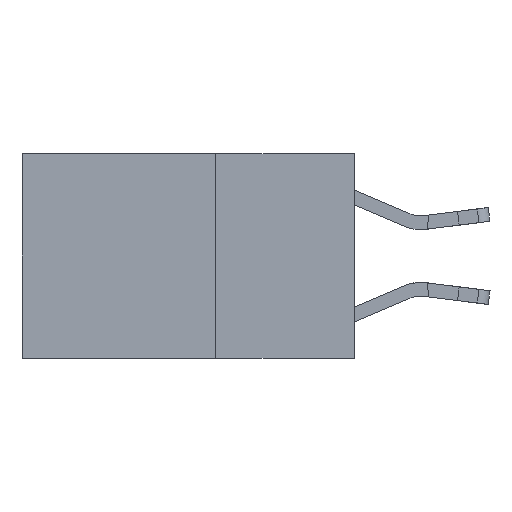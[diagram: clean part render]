
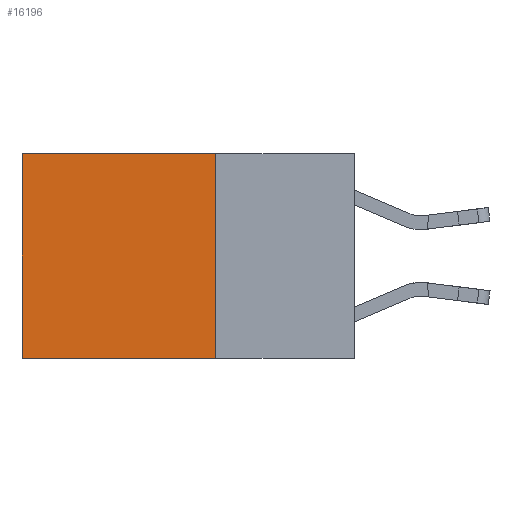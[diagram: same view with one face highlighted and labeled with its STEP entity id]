
A CAD part, left-side view. The second image highlights one B-rep face of the part: STEP entity #16196.
In plain terms, the highlighted planar face has unit normal (-1, 0, 0).
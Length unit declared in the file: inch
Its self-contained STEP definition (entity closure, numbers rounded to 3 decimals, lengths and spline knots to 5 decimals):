
#192 = ORIENTED_EDGE ( 'NONE', *, *, #11985, .F. ) ;
#1448 = CARTESIAN_POINT ( 'NONE',  ( 0.2625, 0.25, 0. ) ) ;
#2499 = VECTOR ( 'NONE', #9625, 39.37008 ) ;
#2545 = CARTESIAN_POINT ( 'NONE',  ( 0.2625, 0.25, 0. ) ) ;
#2577 = VECTOR ( 'NONE', #10538, 39.37008 ) ;
#2944 = ORIENTED_EDGE ( 'NONE', *, *, #8381, .T. ) ;
#3586 = CARTESIAN_POINT ( 'NONE',  ( 0.2625, 0.6, 0. ) ) ;
#3751 = CARTESIAN_POINT ( 'NONE',  ( 0.2625, 0.25, -0.37 ) ) ;
#3817 = PLANE ( 'NONE',  #12852 ) ;
#4445 = CARTESIAN_POINT ( 'NONE',  ( 0.2625, 0.6, -0.37 ) ) ;
#4901 = LINE ( 'NONE', #14994, #2499 ) ;
#5001 = VERTEX_POINT ( 'NONE', #1448 ) ;
#5248 = EDGE_CURVE ( 'NONE', #8953, #6464, #11733, .T. ) ;
#5282 = VERTEX_POINT ( 'NONE', #3586 ) ;
#5364 = DIRECTION ( 'NONE',  ( 1., 0., 0. ) ) ;
#5477 = CARTESIAN_POINT ( 'NONE',  ( 0.2625, 0.25, -0.37 ) ) ;
#5478 = CARTESIAN_POINT ( 'NONE',  ( 0.2625, 0.25, 0. ) ) ;
#5893 = LINE ( 'NONE', #8606, #17463 ) ;
#6464 = VERTEX_POINT ( 'NONE', #4445 ) ;
#8283 = ORIENTED_EDGE ( 'NONE', *, *, #15289, .T. ) ;
#8381 = EDGE_CURVE ( 'NONE', #5282, #6464, #4901, .T. ) ;
#8553 = DIRECTION ( 'NONE',  ( 0., 0., -1. ) ) ;
#8606 = CARTESIAN_POINT ( 'NONE',  ( 0.2625, 0.25, 0. ) ) ;
#8953 = VERTEX_POINT ( 'NONE', #5477 ) ;
#9625 = DIRECTION ( 'NONE',  ( 0., 0., -1. ) ) ;
#10144 = EDGE_LOOP ( 'NONE', ( #2944, #10483, #192, #8283 ) ) ;
#10483 = ORIENTED_EDGE ( 'NONE', *, *, #5248, .F. ) ;
#10538 = DIRECTION ( 'NONE',  ( 0., 1., 0. ) ) ;
#11733 = LINE ( 'NONE', #3751, #2577 ) ;
#11985 = EDGE_CURVE ( 'NONE', #5001, #8953, #5893, .T. ) ;
#12099 = FACE_OUTER_BOUND ( 'NONE', #10144, .T. ) ;
#12852 = AXIS2_PLACEMENT_3D ( 'NONE', #2545, #5364, #17738 ) ;
#14994 = CARTESIAN_POINT ( 'NONE',  ( 0.2625, 0.6, 0. ) ) ;
#15226 = DIRECTION ( 'NONE',  ( 0., 1., 0. ) ) ;
#15289 = EDGE_CURVE ( 'NONE', #5001, #5282, #15859, .T. ) ;
#15859 = LINE ( 'NONE', #5478, #16088 ) ;
#16088 = VECTOR ( 'NONE', #15226, 39.37008 ) ;
#16196 = ADVANCED_FACE ( 'NONE', ( #12099 ), #3817, .F. ) ;
#17463 = VECTOR ( 'NONE', #8553, 39.37008 ) ;
#17738 = DIRECTION ( 'NONE',  ( 0., 0., -1. ) ) ;
